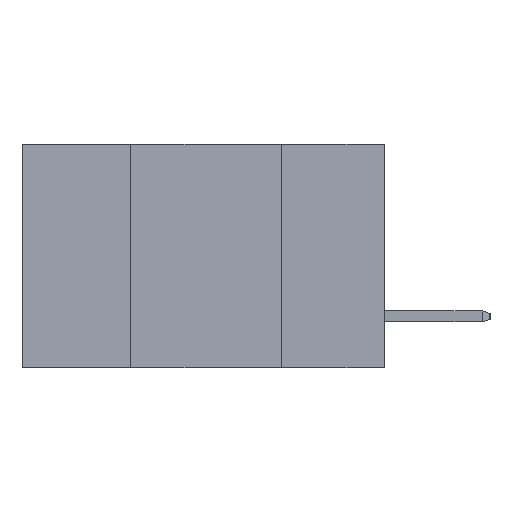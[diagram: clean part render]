
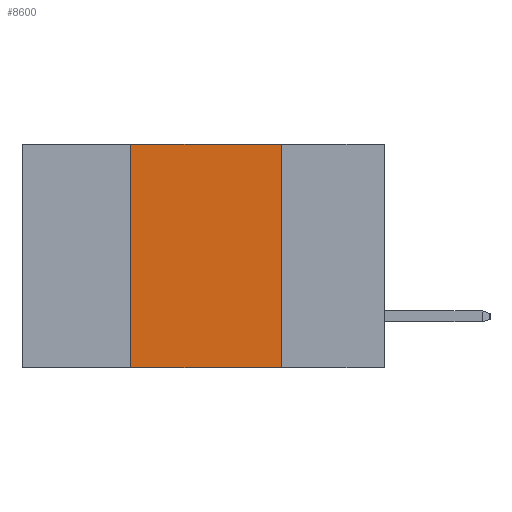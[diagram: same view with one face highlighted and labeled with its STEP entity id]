
A CAD part, left-side view. The second image highlights one B-rep face of the part: STEP entity #8600.
In plain terms, the highlighted planar face has unit normal (-1, 0, 0).
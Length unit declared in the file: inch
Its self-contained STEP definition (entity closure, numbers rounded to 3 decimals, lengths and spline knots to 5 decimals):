
#306 = LINE ( 'NONE', #8928, #9830 ) ;
#376 = DIRECTION ( 'NONE',  ( 1., 0., 0. ) ) ;
#756 = DIRECTION ( 'NONE',  ( 0., -1., 0. ) ) ;
#827 = CARTESIAN_POINT ( 'NONE',  ( 0., 0.42, 0. ) ) ;
#1211 = VECTOR ( 'NONE', #6258, 39.37008 ) ;
#1527 = EDGE_CURVE ( 'NONE', #7260, #5634, #306, .T. ) ;
#1682 = CARTESIAN_POINT ( 'NONE',  ( 0., 0.6, 0. ) ) ;
#1860 = CARTESIAN_POINT ( 'NONE',  ( 0., 0.42, -0.37 ) ) ;
#2473 = VECTOR ( 'NONE', #756, 39.37008 ) ;
#2522 = EDGE_CURVE ( 'NONE', #2653, #7260, #10739, .T. ) ;
#2562 = CARTESIAN_POINT ( 'NONE',  ( 0., 0.42, 0. ) ) ;
#2653 = VERTEX_POINT ( 'NONE', #827 ) ;
#3811 = LINE ( 'NONE', #2562, #1211 ) ;
#4355 = EDGE_LOOP ( 'NONE', ( #8281, #5938, #4526, #9514 ) ) ;
#4526 = ORIENTED_EDGE ( 'NONE', *, *, #8750, .F. ) ;
#5021 = LINE ( 'NONE', #10777, #2473 ) ;
#5186 = PLANE ( 'NONE',  #9821 ) ;
#5634 = VERTEX_POINT ( 'NONE', #8681 ) ;
#5938 = ORIENTED_EDGE ( 'NONE', *, *, #2522, .F. ) ;
#6070 = VECTOR ( 'NONE', #8782, 39.37008 ) ;
#6258 = DIRECTION ( 'NONE',  ( 0., 0., 1. ) ) ;
#6981 = DIRECTION ( 'NONE',  ( 0., 0., -1. ) ) ;
#6998 = EDGE_CURVE ( 'NONE', #7719, #5634, #5021, .T. ) ;
#7260 = VERTEX_POINT ( 'NONE', #8566 ) ;
#7719 = VERTEX_POINT ( 'NONE', #1860 ) ;
#7895 = FACE_OUTER_BOUND ( 'NONE', #4355, .T. ) ;
#8281 = ORIENTED_EDGE ( 'NONE', *, *, #1527, .F. ) ;
#8566 = CARTESIAN_POINT ( 'NONE',  ( 0., 0.17, 0. ) ) ;
#8600 = ADVANCED_FACE ( 'NONE', ( #7895 ), #5186, .F. ) ;
#8681 = CARTESIAN_POINT ( 'NONE',  ( 0., 0.17, -0.37 ) ) ;
#8750 = EDGE_CURVE ( 'NONE', #7719, #2653, #3811, .T. ) ;
#8782 = DIRECTION ( 'NONE',  ( 0., -1., 0. ) ) ;
#8928 = CARTESIAN_POINT ( 'NONE',  ( 0., 0.17, 0. ) ) ;
#9097 = DIRECTION ( 'NONE',  ( 0., 0., -1. ) ) ;
#9514 = ORIENTED_EDGE ( 'NONE', *, *, #6998, .T. ) ;
#9573 = CARTESIAN_POINT ( 'NONE',  ( 0., 0.6, 0. ) ) ;
#9821 = AXIS2_PLACEMENT_3D ( 'NONE', #9573, #376, #6981 ) ;
#9830 = VECTOR ( 'NONE', #9097, 39.37008 ) ;
#10739 = LINE ( 'NONE', #1682, #6070 ) ;
#10777 = CARTESIAN_POINT ( 'NONE',  ( 0., 0.6, -0.37 ) ) ;
